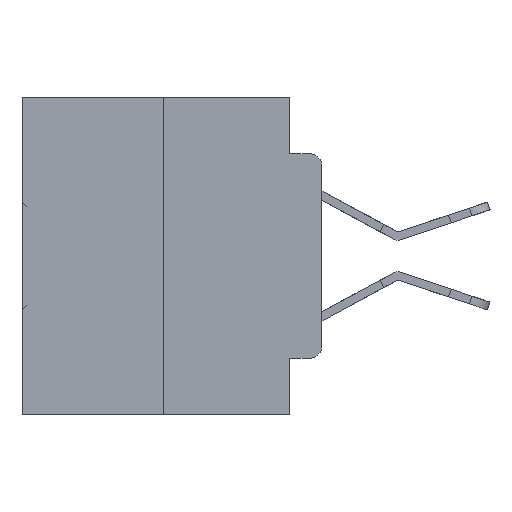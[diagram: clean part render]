
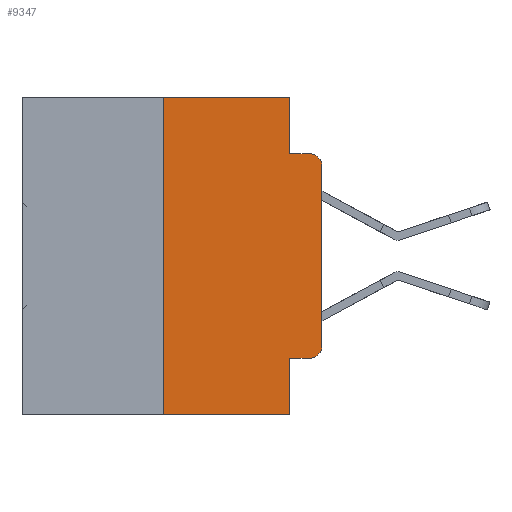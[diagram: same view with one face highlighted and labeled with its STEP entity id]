
A CAD part, left-side view. The second image highlights one B-rep face of the part: STEP entity #9347.
In plain terms, the highlighted planar face has unit normal (-1, 0, 0).
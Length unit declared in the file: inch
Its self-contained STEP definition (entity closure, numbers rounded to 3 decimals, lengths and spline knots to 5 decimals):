
#1002 = VERTEX_POINT ( 'NONE', #10445 ) ;
#1250 = VECTOR ( 'NONE', #26730, 39.37008 ) ;
#2002 = CARTESIAN_POINT ( 'NONE',  ( 0., 0.473, 0. ) ) ;
#2534 = DIRECTION ( 'NONE',  ( 0., -1., 0. ) ) ;
#2675 = ORIENTED_EDGE ( 'NONE', *, *, #26103, .F. ) ;
#2873 = EDGE_CURVE ( 'NONE', #15507, #10579, #10523, .T. ) ;
#3707 = VECTOR ( 'NONE', #34607, 39.37008 ) ;
#4108 = ORIENTED_EDGE ( 'NONE', *, *, #22839, .T. ) ;
#4118 = DIRECTION ( 'NONE',  ( 0., -1., 0. ) ) ;
#4237 = DIRECTION ( 'NONE',  ( -1., 0., 0. ) ) ;
#4363 = EDGE_LOOP ( 'NONE', ( #4108, #29500, #4381, #6613, #2675, #8264, #29801, #4695, #26887, #25872 ) ) ;
#4381 = ORIENTED_EDGE ( 'NONE', *, *, #32448, .F. ) ;
#4560 = EDGE_CURVE ( 'NONE', #5475, #22681, #20324, .T. ) ;
#4695 = ORIENTED_EDGE ( 'NONE', *, *, #2873, .F. ) ;
#5065 = LINE ( 'NONE', #21265, #17209 ) ;
#5475 = VERTEX_POINT ( 'NONE', #35441 ) ;
#6613 = ORIENTED_EDGE ( 'NONE', *, *, #22484, .F. ) ;
#7552 = VERTEX_POINT ( 'NONE', #17292 ) ;
#8264 = ORIENTED_EDGE ( 'NONE', *, *, #10648, .F. ) ;
#8318 = AXIS2_PLACEMENT_3D ( 'NONE', #12230, #20518, #28792 ) ;
#8554 = LINE ( 'NONE', #22406, #16416 ) ;
#9347 = ADVANCED_FACE ( 'NONE', ( #35489 ), #19263, .F. ) ;
#9472 = VERTEX_POINT ( 'NONE', #15244 ) ;
#10445 = CARTESIAN_POINT ( 'NONE',  ( 0., 0., -0.1085 ) ) ;
#10523 = LINE ( 'NONE', #30147, #1250 ) ;
#10579 = VERTEX_POINT ( 'NONE', #24310 ) ;
#10648 = EDGE_CURVE ( 'NONE', #7552, #9472, #5065, .T. ) ;
#10841 = VERTEX_POINT ( 'NONE', #14778 ) ;
#11535 = CARTESIAN_POINT ( 'NONE',  ( 0., 0., 0. ) ) ;
#11746 = LINE ( 'NONE', #22919, #33573 ) ;
#11805 = VERTEX_POINT ( 'NONE', #16427 ) ;
#12230 = CARTESIAN_POINT ( 'NONE',  ( 0., 0.02, -0.1085 ) ) ;
#14291 = EDGE_CURVE ( 'NONE', #7552, #10579, #28673, .T. ) ;
#14778 = CARTESIAN_POINT ( 'NONE',  ( 0., 0.02, -0.0885 ) ) ;
#15244 = CARTESIAN_POINT ( 'NONE',  ( 0., 0.25, 0. ) ) ;
#15507 = VERTEX_POINT ( 'NONE', #31167 ) ;
#16056 = DIRECTION ( 'NONE',  ( 0., 0., 1. ) ) ;
#16416 = VECTOR ( 'NONE', #33396, 39.37008 ) ;
#16427 = CARTESIAN_POINT ( 'NONE',  ( 0., 0.051, -0.0885 ) ) ;
#16556 = AXIS2_PLACEMENT_3D ( 'NONE', #19622, #16758, #25221 ) ;
#16758 = DIRECTION ( 'NONE',  ( 1., 0., 0. ) ) ;
#17209 = VECTOR ( 'NONE', #16056, 39.37008 ) ;
#17292 = CARTESIAN_POINT ( 'NONE',  ( 0., 0.25, -0.5 ) ) ;
#17652 = LINE ( 'NONE', #11535, #31310 ) ;
#18038 = CARTESIAN_POINT ( 'NONE',  ( 0., 0.473, -0.5 ) ) ;
#18307 = CARTESIAN_POINT ( 'NONE',  ( 0., 0.02, -0.3915 ) ) ;
#18828 = VECTOR ( 'NONE', #2534, 39.37008 ) ;
#19263 = PLANE ( 'NONE',  #16556 ) ;
#19622 = CARTESIAN_POINT ( 'NONE',  ( 0., 0.473, 0. ) ) ;
#20207 = DIRECTION ( 'NONE',  ( 0., 0., -1. ) ) ;
#20324 = CIRCLE ( 'NONE', #24356, 0.02 ) ;
#20518 = DIRECTION ( 'NONE',  ( -1., 0., 0. ) ) ;
#20569 = VECTOR ( 'NONE', #4118, 39.37008 ) ;
#21265 = CARTESIAN_POINT ( 'NONE',  ( 0., 0.25, 0. ) ) ;
#22406 = CARTESIAN_POINT ( 'NONE',  ( 0., 0.051, -0.4115 ) ) ;
#22484 = EDGE_CURVE ( 'NONE', #33308, #11805, #11746, .T. ) ;
#22681 = VERTEX_POINT ( 'NONE', #32965 ) ;
#22839 = EDGE_CURVE ( 'NONE', #22681, #1002, #17652, .T. ) ;
#22919 = CARTESIAN_POINT ( 'NONE',  ( 0., 0.051, 0. ) ) ;
#23147 = EDGE_CURVE ( 'NONE', #1002, #10841, #26715, .T. ) ;
#23221 = CARTESIAN_POINT ( 'NONE',  ( 0., 0.051, -0.0885 ) ) ;
#24310 = CARTESIAN_POINT ( 'NONE',  ( 0., 0.051, -0.5 ) ) ;
#24356 = AXIS2_PLACEMENT_3D ( 'NONE', #18307, #4237, #35207 ) ;
#24467 = EDGE_CURVE ( 'NONE', #15507, #5475, #8554, .T. ) ;
#25221 = DIRECTION ( 'NONE',  ( 0., 0., -1. ) ) ;
#25554 = DIRECTION ( 'NONE',  ( 0., 0., 1. ) ) ;
#25872 = ORIENTED_EDGE ( 'NONE', *, *, #4560, .T. ) ;
#25916 = LINE ( 'NONE', #23221, #20569 ) ;
#26103 = EDGE_CURVE ( 'NONE', #9472, #33308, #29387, .T. ) ;
#26715 = CIRCLE ( 'NONE', #8318, 0.02 ) ;
#26730 = DIRECTION ( 'NONE',  ( 0., 0., -1. ) ) ;
#26887 = ORIENTED_EDGE ( 'NONE', *, *, #24467, .T. ) ;
#28673 = LINE ( 'NONE', #18038, #3707 ) ;
#28792 = DIRECTION ( 'NONE',  ( 0., 0., -1. ) ) ;
#29387 = LINE ( 'NONE', #2002, #18828 ) ;
#29500 = ORIENTED_EDGE ( 'NONE', *, *, #23147, .T. ) ;
#29801 = ORIENTED_EDGE ( 'NONE', *, *, #14291, .T. ) ;
#30147 = CARTESIAN_POINT ( 'NONE',  ( 0., 0.051, 0. ) ) ;
#31091 = CARTESIAN_POINT ( 'NONE',  ( 0., 0.051, 0. ) ) ;
#31167 = CARTESIAN_POINT ( 'NONE',  ( 0., 0.051, -0.4115 ) ) ;
#31310 = VECTOR ( 'NONE', #25554, 39.37008 ) ;
#32448 = EDGE_CURVE ( 'NONE', #11805, #10841, #25916, .T. ) ;
#32965 = CARTESIAN_POINT ( 'NONE',  ( 0., 0., -0.3915 ) ) ;
#33308 = VERTEX_POINT ( 'NONE', #31091 ) ;
#33396 = DIRECTION ( 'NONE',  ( 0., -1., 0. ) ) ;
#33573 = VECTOR ( 'NONE', #20207, 39.37008 ) ;
#34607 = DIRECTION ( 'NONE',  ( 0., -1., 0. ) ) ;
#35207 = DIRECTION ( 'NONE',  ( 0., 0., -1. ) ) ;
#35441 = CARTESIAN_POINT ( 'NONE',  ( 0., 0.02, -0.4115 ) ) ;
#35489 = FACE_OUTER_BOUND ( 'NONE', #4363, .T. ) ;
